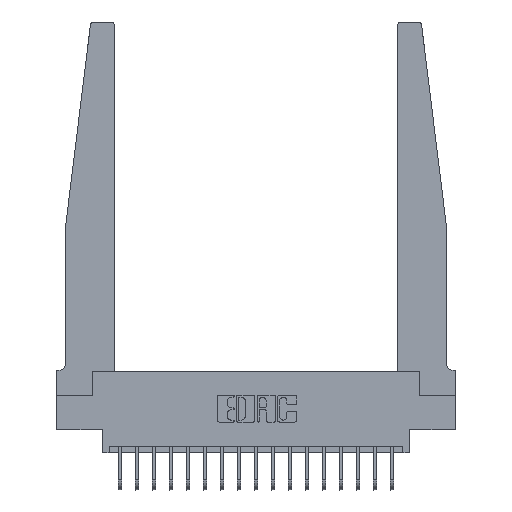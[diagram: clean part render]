
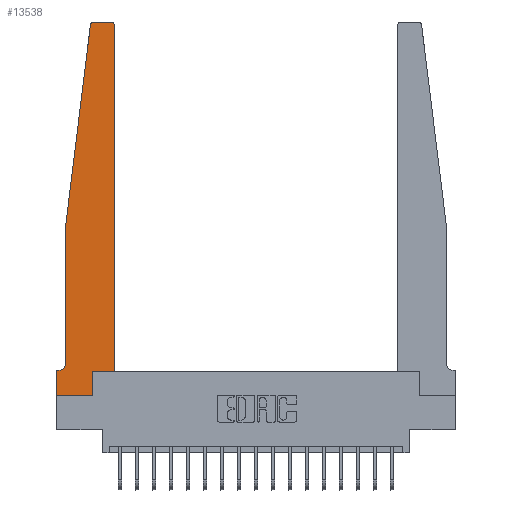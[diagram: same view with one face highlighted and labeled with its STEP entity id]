
A CAD part, top view. The second image highlights one B-rep face of the part: STEP entity #13538.
In plain terms, the highlighted planar face has unit normal (0, 0, 1).
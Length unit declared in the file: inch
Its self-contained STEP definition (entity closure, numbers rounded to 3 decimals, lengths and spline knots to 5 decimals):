
#355 = DIRECTION ( 'NONE',  ( 1., 0., 0. ) ) ;
#411 = DIRECTION ( 'NONE',  ( 1., 0., 0. ) ) ;
#515 = LINE ( 'NONE', #13941, #4515 ) ;
#637 = DIRECTION ( 'NONE',  ( 0., 0., -1. ) ) ;
#1042 = DIRECTION ( 'NONE',  ( 0., -1., 0. ) ) ;
#1210 = DIRECTION ( 'NONE',  ( 0., 1., 0. ) ) ;
#1297 = CARTESIAN_POINT ( 'NONE',  ( 0.425, 0.18, 0.37 ) ) ;
#1346 = ORIENTED_EDGE ( 'NONE', *, *, #9196, .T. ) ;
#1684 = VERTEX_POINT ( 'NONE', #8709 ) ;
#1774 = VERTEX_POINT ( 'NONE', #10265 ) ;
#1872 = EDGE_CURVE ( 'NONE', #13720, #18363, #16939, .T. ) ;
#1895 = CIRCLE ( 'NONE', #3765, 0.03 ) ;
#2115 = CARTESIAN_POINT ( 'NONE',  ( 0.2605, 0.18, 0.37 ) ) ;
#2118 = CARTESIAN_POINT ( 'NONE',  ( 0., 0.1875, 0.37 ) ) ;
#2232 = ORIENTED_EDGE ( 'NONE', *, *, #16132, .T. ) ;
#2419 = EDGE_LOOP ( 'NONE', ( #2232, #3842, #17718, #10271, #13158, #7965, #11425, #13311, #11823, #11723, #9478, #1346 ) ) ;
#3119 = VECTOR ( 'NONE', #16669, 39.37008 ) ;
#3167 = DIRECTION ( 'NONE',  ( 1., 0., 0. ) ) ;
#3458 = DIRECTION ( 'NONE',  ( -1., 0., 0. ) ) ;
#3529 = VERTEX_POINT ( 'NONE', #15302 ) ;
#3575 = CARTESIAN_POINT ( 'NONE',  ( 0.015, 0.2375, 0.37 ) ) ;
#3672 = CARTESIAN_POINT ( 'NONE',  ( 0.425, 2.72, 0.37 ) ) ;
#3765 = AXIS2_PLACEMENT_3D ( 'NONE', #6712, #14150, #11011 ) ;
#3772 = CARTESIAN_POINT ( 'NONE',  ( 0., 0., 0.37 ) ) ;
#3842 = ORIENTED_EDGE ( 'NONE', *, *, #6751, .T. ) ;
#3968 = PLANE ( 'NONE',  #7046 ) ;
#4135 = VERTEX_POINT ( 'NONE', #10433 ) ;
#4440 = VERTEX_POINT ( 'NONE', #14558 ) ;
#4515 = VECTOR ( 'NONE', #3458, 39.37008 ) ;
#4687 = CARTESIAN_POINT ( 'NONE',  ( 0., 0., 0.37 ) ) ;
#4721 = LINE ( 'NONE', #10681, #3119 ) ;
#5164 = CARTESIAN_POINT ( 'NONE',  ( 0.065, 1.25, 0.37 ) ) ;
#5216 = AXIS2_PLACEMENT_3D ( 'NONE', #3575, #637, #18754 ) ;
#5267 = VECTOR ( 'NONE', #1210, 39.37008 ) ;
#5473 = VERTEX_POINT ( 'NONE', #7805 ) ;
#5651 = LINE ( 'NONE', #17204, #18078 ) ;
#6144 = VECTOR ( 'NONE', #3167, 39.37008 ) ;
#6397 = VECTOR ( 'NONE', #411, 39.37008 ) ;
#6544 = DIRECTION ( 'NONE',  ( 0., 0., 1. ) ) ;
#6712 = CARTESIAN_POINT ( 'NONE',  ( 0.395, 2.72, 0.37 ) ) ;
#6751 = EDGE_CURVE ( 'NONE', #1774, #13846, #16831, .T. ) ;
#6833 = DIRECTION ( 'NONE',  ( -0.122, -0.992, 0. ) ) ;
#6992 = VECTOR ( 'NONE', #10853, 39.37008 ) ;
#7046 = AXIS2_PLACEMENT_3D ( 'NONE', #2118, #8087, #14252 ) ;
#7805 = CARTESIAN_POINT ( 'NONE',  ( 0.2605, 0., 0.37 ) ) ;
#7863 = CARTESIAN_POINT ( 'NONE',  ( 0.24675, 2.72367, 0.37 ) ) ;
#7902 = LINE ( 'NONE', #18178, #18402 ) ;
#7964 = EDGE_CURVE ( 'NONE', #5473, #12435, #4721, .T. ) ;
#7965 = ORIENTED_EDGE ( 'NONE', *, *, #18469, .T. ) ;
#8087 = DIRECTION ( 'NONE',  ( 0., 0., 1. ) ) ;
#8286 = LINE ( 'NONE', #5164, #18258 ) ;
#8709 = CARTESIAN_POINT ( 'NONE',  ( 0.395, 2.75, 0.37 ) ) ;
#9084 = DIRECTION ( 'NONE',  ( -1., 0., 0. ) ) ;
#9196 = EDGE_CURVE ( 'NONE', #13571, #1684, #1895, .T. ) ;
#9236 = LINE ( 'NONE', #11088, #6397 ) ;
#9286 = CARTESIAN_POINT ( 'NONE',  ( 0.27653, 2.72, 0.37 ) ) ;
#9478 = ORIENTED_EDGE ( 'NONE', *, *, #18595, .T. ) ;
#10265 = CARTESIAN_POINT ( 'NONE',  ( 0.27653, 2.75, 0.37 ) ) ;
#10271 = ORIENTED_EDGE ( 'NONE', *, *, #18326, .T. ) ;
#10433 = CARTESIAN_POINT ( 'NONE',  ( 0.015, 0.1875, 0.37 ) ) ;
#10510 = CIRCLE ( 'NONE', #5216, 0.05 ) ;
#10681 = CARTESIAN_POINT ( 'NONE',  ( 0.2605, 0.18, 0.37 ) ) ;
#10853 = DIRECTION ( 'NONE',  ( 0., -1., 0. ) ) ;
#11011 = DIRECTION ( 'NONE',  ( 1., 0., 0. ) ) ;
#11088 = CARTESIAN_POINT ( 'NONE',  ( 0.425, 0.18, 0.37 ) ) ;
#11425 = ORIENTED_EDGE ( 'NONE', *, *, #1872, .T. ) ;
#11723 = ORIENTED_EDGE ( 'NONE', *, *, #16200, .T. ) ;
#11823 = ORIENTED_EDGE ( 'NONE', *, *, #7964, .T. ) ;
#11895 = VERTEX_POINT ( 'NONE', #13987 ) ;
#12026 = EDGE_CURVE ( 'NONE', #13846, #3529, #8286, .T. ) ;
#12435 = VERTEX_POINT ( 'NONE', #2115 ) ;
#13158 = ORIENTED_EDGE ( 'NONE', *, *, #17679, .T. ) ;
#13311 = ORIENTED_EDGE ( 'NONE', *, *, #17884, .T. ) ;
#13538 = ADVANCED_FACE ( 'NONE', ( #15531 ), #3968, .T. ) ;
#13571 = VERTEX_POINT ( 'NONE', #3672 ) ;
#13720 = VERTEX_POINT ( 'NONE', #19213 ) ;
#13846 = VERTEX_POINT ( 'NONE', #7863 ) ;
#13941 = CARTESIAN_POINT ( 'NONE',  ( 0.25, 2.75, 0.37 ) ) ;
#13987 = CARTESIAN_POINT ( 'NONE',  ( 0.065, 0.2375, 0.37 ) ) ;
#14150 = DIRECTION ( 'NONE',  ( 0., 0., 1. ) ) ;
#14252 = DIRECTION ( 'NONE',  ( 1., 0., 0. ) ) ;
#14558 = CARTESIAN_POINT ( 'NONE',  ( 0.425, 0.18, 0.37 ) ) ;
#14729 = LINE ( 'NONE', #1297, #5267 ) ;
#15302 = CARTESIAN_POINT ( 'NONE',  ( 0.065, 1.25, 0.37 ) ) ;
#15531 = FACE_OUTER_BOUND ( 'NONE', #2419, .T. ) ;
#15885 = AXIS2_PLACEMENT_3D ( 'NONE', #9286, #6544, #355 ) ;
#16132 = EDGE_CURVE ( 'NONE', #1684, #1774, #515, .T. ) ;
#16200 = EDGE_CURVE ( 'NONE', #12435, #4440, #9236, .T. ) ;
#16583 = LINE ( 'NONE', #16792, #6144 ) ;
#16669 = DIRECTION ( 'NONE',  ( 0., 1., 0. ) ) ;
#16792 = CARTESIAN_POINT ( 'NONE',  ( 0., 0., 0.37 ) ) ;
#16831 = CIRCLE ( 'NONE', #15885, 0.03 ) ;
#16939 = LINE ( 'NONE', #4687, #6992 ) ;
#17204 = CARTESIAN_POINT ( 'NONE',  ( 0.065, 1.25, 0.37 ) ) ;
#17679 = EDGE_CURVE ( 'NONE', #11895, #4135, #10510, .T. ) ;
#17718 = ORIENTED_EDGE ( 'NONE', *, *, #12026, .T. ) ;
#17884 = EDGE_CURVE ( 'NONE', #18363, #5473, #16583, .T. ) ;
#18078 = VECTOR ( 'NONE', #1042, 39.37008 ) ;
#18178 = CARTESIAN_POINT ( 'NONE',  ( 0.065, 0.1875, 0.37 ) ) ;
#18258 = VECTOR ( 'NONE', #6833, 39.37008 ) ;
#18326 = EDGE_CURVE ( 'NONE', #3529, #11895, #5651, .T. ) ;
#18363 = VERTEX_POINT ( 'NONE', #3772 ) ;
#18402 = VECTOR ( 'NONE', #9084, 39.37008 ) ;
#18469 = EDGE_CURVE ( 'NONE', #4135, #13720, #7902, .T. ) ;
#18595 = EDGE_CURVE ( 'NONE', #4440, #13571, #14729, .T. ) ;
#18754 = DIRECTION ( 'NONE',  ( -1., 0., 0. ) ) ;
#19213 = CARTESIAN_POINT ( 'NONE',  ( 0., 0.1875, 0.37 ) ) ;
